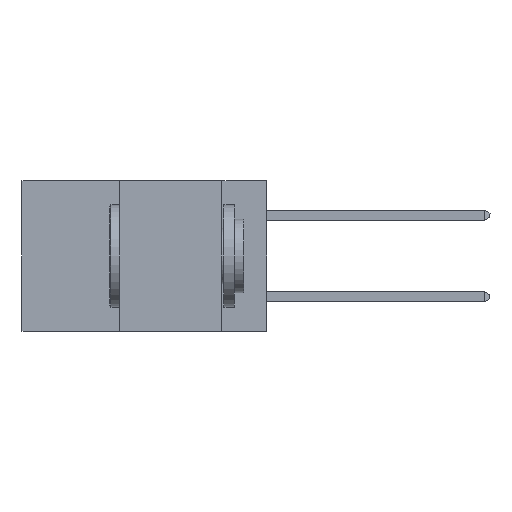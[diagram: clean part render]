
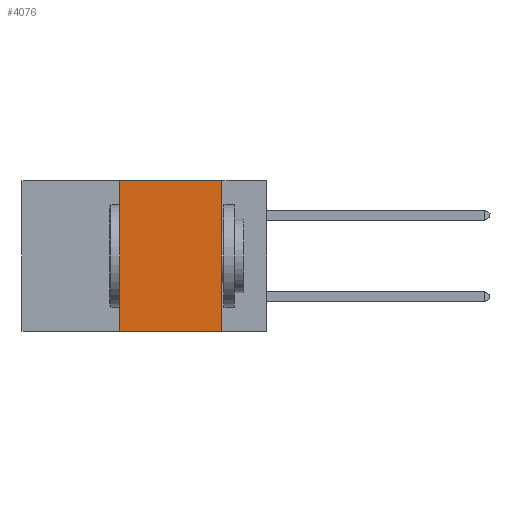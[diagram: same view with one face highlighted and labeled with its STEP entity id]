
A CAD part, left-side view. The second image highlights one B-rep face of the part: STEP entity #4076.
In plain terms, the highlighted planar face has unit normal (-1, 0, 0).
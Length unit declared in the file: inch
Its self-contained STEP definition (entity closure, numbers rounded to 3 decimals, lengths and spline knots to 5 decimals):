
#123 = VERTEX_POINT ( 'NONE', #2756 ) ;
#208 = AXIS2_PLACEMENT_3D ( 'NONE', #5626, #5126, #5039 ) ;
#1136 = VECTOR ( 'NONE', #3118, 39.37008 ) ;
#1164 = DIRECTION ( 'NONE',  ( 0., 0., 1. ) ) ;
#1181 = CARTESIAN_POINT ( 'NONE',  ( 0., 0.36, 0. ) ) ;
#1451 = VECTOR ( 'NONE', #4515, 39.37008 ) ;
#1501 = EDGE_CURVE ( 'NONE', #123, #7992, #8706, .T. ) ;
#1732 = ORIENTED_EDGE ( 'NONE', *, *, #1501, .F. ) ;
#2329 = VERTEX_POINT ( 'NONE', #7303 ) ;
#2586 = CARTESIAN_POINT ( 'NONE',  ( 0., 0.11, 0. ) ) ;
#2756 = CARTESIAN_POINT ( 'NONE',  ( 0., 0.36, -0.37 ) ) ;
#2920 = EDGE_CURVE ( 'NONE', #7992, #4695, #7469, .T. ) ;
#3118 = DIRECTION ( 'NONE',  ( 0., 0., -1. ) ) ;
#3328 = LINE ( 'NONE', #6787, #1136 ) ;
#3375 = FACE_OUTER_BOUND ( 'NONE', #7334, .T. ) ;
#4076 = ADVANCED_FACE ( 'NONE', ( #3375 ), #4557, .F. ) ;
#4515 = DIRECTION ( 'NONE',  ( 0., -1., 0. ) ) ;
#4528 = CARTESIAN_POINT ( 'NONE',  ( 0., 0.6, 0. ) ) ;
#4557 = PLANE ( 'NONE',  #208 ) ;
#4695 = VERTEX_POINT ( 'NONE', #2586 ) ;
#5039 = DIRECTION ( 'NONE',  ( 0., 0., -1. ) ) ;
#5126 = DIRECTION ( 'NONE',  ( 1., 0., 0. ) ) ;
#5626 = CARTESIAN_POINT ( 'NONE',  ( 0., 0.6, 0. ) ) ;
#5881 = CARTESIAN_POINT ( 'NONE',  ( 0., 0.36, 0. ) ) ;
#6116 = EDGE_CURVE ( 'NONE', #4695, #2329, #3328, .T. ) ;
#6127 = CARTESIAN_POINT ( 'NONE',  ( 0., 0.6, -0.37 ) ) ;
#6787 = CARTESIAN_POINT ( 'NONE',  ( 0., 0.11, 0. ) ) ;
#6845 = DIRECTION ( 'NONE',  ( 0., -1., 0. ) ) ;
#7303 = CARTESIAN_POINT ( 'NONE',  ( 0., 0.11, -0.37 ) ) ;
#7334 = EDGE_LOOP ( 'NONE', ( #9707, #9516, #1732, #9696 ) ) ;
#7469 = LINE ( 'NONE', #4528, #1451 ) ;
#7992 = VERTEX_POINT ( 'NONE', #5881 ) ;
#8706 = LINE ( 'NONE', #1181, #9112 ) ;
#8898 = EDGE_CURVE ( 'NONE', #123, #2329, #9226, .T. ) ;
#9014 = VECTOR ( 'NONE', #6845, 39.37008 ) ;
#9112 = VECTOR ( 'NONE', #1164, 39.37008 ) ;
#9226 = LINE ( 'NONE', #6127, #9014 ) ;
#9516 = ORIENTED_EDGE ( 'NONE', *, *, #2920, .F. ) ;
#9696 = ORIENTED_EDGE ( 'NONE', *, *, #8898, .T. ) ;
#9707 = ORIENTED_EDGE ( 'NONE', *, *, #6116, .F. ) ;
